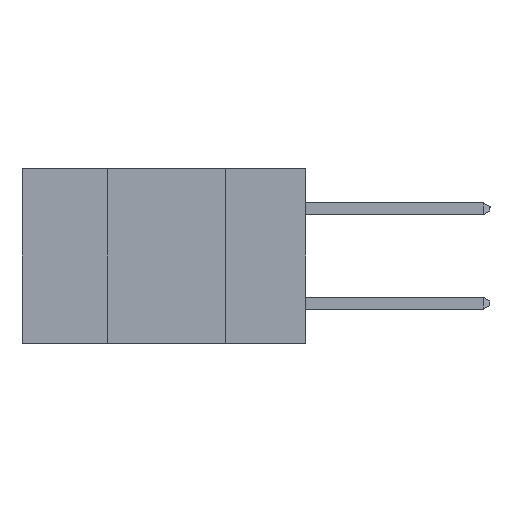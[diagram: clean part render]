
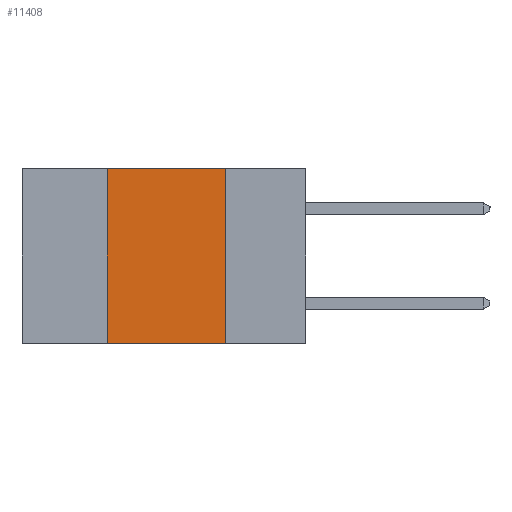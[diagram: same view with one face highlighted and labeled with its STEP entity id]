
A CAD part, left-side view. The second image highlights one B-rep face of the part: STEP entity #11408.
In plain terms, the highlighted planar face has unit normal (-1, 0, 0).
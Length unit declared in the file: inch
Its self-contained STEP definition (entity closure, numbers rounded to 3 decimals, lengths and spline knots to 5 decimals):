
#165 = LINE ( 'NONE', #8553, #14117 ) ;
#1283 = EDGE_CURVE ( 'NONE', #1421, #11434, #5335, .T. ) ;
#1421 = VERTEX_POINT ( 'NONE', #15532 ) ;
#1751 = ORIENTED_EDGE ( 'NONE', *, *, #3717, .T. ) ;
#2440 = FACE_OUTER_BOUND ( 'NONE', #8507, .T. ) ;
#2951 = VERTEX_POINT ( 'NONE', #9743 ) ;
#3098 = LINE ( 'NONE', #4231, #8961 ) ;
#3717 = EDGE_CURVE ( 'NONE', #1421, #2951, #6414, .T. ) ;
#4110 = CARTESIAN_POINT ( 'NONE',  ( 0., 0.42, 0. ) ) ;
#4231 = CARTESIAN_POINT ( 'NONE',  ( 0., 0.6, 0. ) ) ;
#4358 = CARTESIAN_POINT ( 'NONE',  ( 0., 0.42, -0.37 ) ) ;
#5008 = EDGE_CURVE ( 'NONE', #15303, #2951, #165, .T. ) ;
#5226 = CARTESIAN_POINT ( 'NONE',  ( 0., 0.6, -0.37 ) ) ;
#5335 = LINE ( 'NONE', #4358, #9034 ) ;
#5971 = EDGE_CURVE ( 'NONE', #11434, #15303, #3098, .T. ) ;
#6414 = LINE ( 'NONE', #5226, #8987 ) ;
#7360 = PLANE ( 'NONE',  #15238 ) ;
#8335 = DIRECTION ( 'NONE',  ( 0., 0., -1. ) ) ;
#8507 = EDGE_LOOP ( 'NONE', ( #15094, #9320, #10665, #1751 ) ) ;
#8553 = CARTESIAN_POINT ( 'NONE',  ( 0., 0.17, -0.37 ) ) ;
#8961 = VECTOR ( 'NONE', #9144, 39.37008 ) ;
#8987 = VECTOR ( 'NONE', #10118, 39.37008 ) ;
#9034 = VECTOR ( 'NONE', #9260, 39.37008 ) ;
#9144 = DIRECTION ( 'NONE',  ( 0., -1., 0. ) ) ;
#9260 = DIRECTION ( 'NONE',  ( 0., 0., 1. ) ) ;
#9320 = ORIENTED_EDGE ( 'NONE', *, *, #5971, .F. ) ;
#9743 = CARTESIAN_POINT ( 'NONE',  ( 0., 0.17, -0.37 ) ) ;
#10118 = DIRECTION ( 'NONE',  ( 0., -1., 0. ) ) ;
#10665 = ORIENTED_EDGE ( 'NONE', *, *, #1283, .F. ) ;
#11408 = ADVANCED_FACE ( 'NONE', ( #2440 ), #7360, .F. ) ;
#11434 = VERTEX_POINT ( 'NONE', #4110 ) ;
#12303 = DIRECTION ( 'NONE',  ( 0., 0., -1. ) ) ;
#12317 = CARTESIAN_POINT ( 'NONE',  ( 0., 0.6, 0. ) ) ;
#13777 = CARTESIAN_POINT ( 'NONE',  ( 0., 0.17, 0. ) ) ;
#14117 = VECTOR ( 'NONE', #12303, 39.37008 ) ;
#14424 = DIRECTION ( 'NONE',  ( 1., 0., 0. ) ) ;
#15094 = ORIENTED_EDGE ( 'NONE', *, *, #5008, .F. ) ;
#15238 = AXIS2_PLACEMENT_3D ( 'NONE', #12317, #14424, #8335 ) ;
#15303 = VERTEX_POINT ( 'NONE', #13777 ) ;
#15532 = CARTESIAN_POINT ( 'NONE',  ( 0., 0.42, -0.37 ) ) ;
